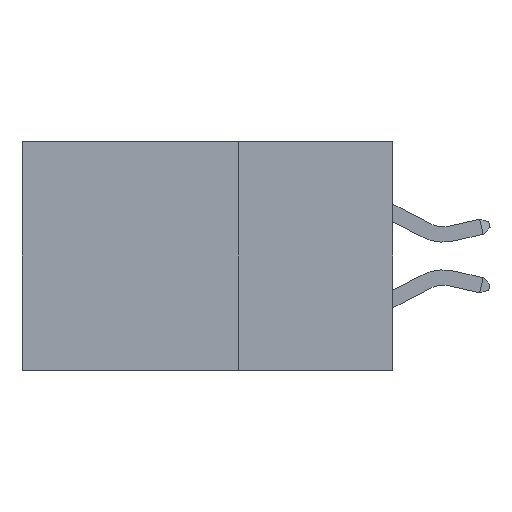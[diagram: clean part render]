
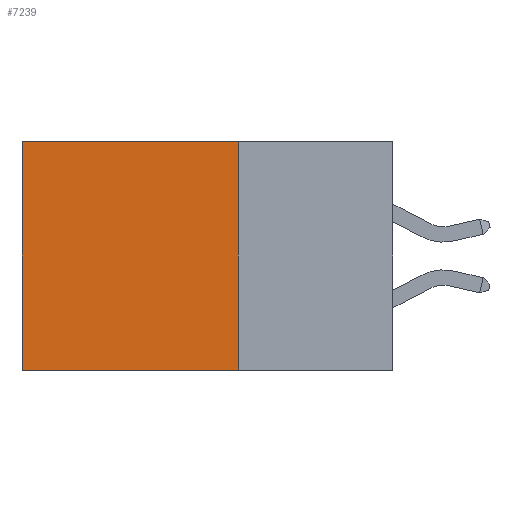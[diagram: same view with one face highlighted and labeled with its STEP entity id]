
A CAD part, left-side view. The second image highlights one B-rep face of the part: STEP entity #7239.
In plain terms, the highlighted planar face has unit normal (-1, 0, 0).
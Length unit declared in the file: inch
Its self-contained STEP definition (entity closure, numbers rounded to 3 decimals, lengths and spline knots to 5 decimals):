
#3 = DIRECTION ( 'NONE',  ( 0., 0., -1. ) ) ;
#237 = VECTOR ( 'NONE', #8397, 39.37008 ) ;
#332 = DIRECTION ( 'NONE',  ( 0., 1., 0. ) ) ;
#712 = DIRECTION ( 'NONE',  ( 0., 0., -1. ) ) ;
#816 = CARTESIAN_POINT ( 'NONE',  ( 0.2875, 0.6, -0.37 ) ) ;
#1140 = EDGE_CURVE ( 'NONE', #10898, #10252, #10301, .T. ) ;
#2216 = VECTOR ( 'NONE', #3, 39.37008 ) ;
#2453 = EDGE_CURVE ( 'NONE', #8843, #10898, #10870, .T. ) ;
#3740 = CARTESIAN_POINT ( 'NONE',  ( 0.2875, 0.25, 0. ) ) ;
#4694 = PLANE ( 'NONE',  #7935 ) ;
#4788 = CARTESIAN_POINT ( 'NONE',  ( 0.2875, 0.25, 0. ) ) ;
#5126 = CARTESIAN_POINT ( 'NONE',  ( 0.2875, 0.25, -0.37 ) ) ;
#5264 = EDGE_CURVE ( 'NONE', #8843, #10979, #7768, .T. ) ;
#5295 = CARTESIAN_POINT ( 'NONE',  ( 0.2875, 0.6, 0. ) ) ;
#5624 = DIRECTION ( 'NONE',  ( 0., 0., -1. ) ) ;
#6026 = CARTESIAN_POINT ( 'NONE',  ( 0.2875, 0.25, 0. ) ) ;
#6212 = CARTESIAN_POINT ( 'NONE',  ( 0.2875, 0.25, -0.37 ) ) ;
#7239 = ADVANCED_FACE ( 'NONE', ( #7722 ), #4694, .F. ) ;
#7722 = FACE_OUTER_BOUND ( 'NONE', #7723, .T. ) ;
#7723 = EDGE_LOOP ( 'NONE', ( #8937, #8780, #8626, #8813 ) ) ;
#7768 = LINE ( 'NONE', #8411, #237 ) ;
#7935 = AXIS2_PLACEMENT_3D ( 'NONE', #3740, #10412, #5624 ) ;
#8102 = VECTOR ( 'NONE', #332, 39.37008 ) ;
#8360 = VECTOR ( 'NONE', #712, 39.37008 ) ;
#8397 = DIRECTION ( 'NONE',  ( 0., 1., 0. ) ) ;
#8411 = CARTESIAN_POINT ( 'NONE',  ( 0.2875, 0.25, 0. ) ) ;
#8626 = ORIENTED_EDGE ( 'NONE', *, *, #2453, .F. ) ;
#8780 = ORIENTED_EDGE ( 'NONE', *, *, #1140, .F. ) ;
#8810 = LINE ( 'NONE', #5295, #8360 ) ;
#8813 = ORIENTED_EDGE ( 'NONE', *, *, #5264, .T. ) ;
#8843 = VERTEX_POINT ( 'NONE', #6026 ) ;
#8937 = ORIENTED_EDGE ( 'NONE', *, *, #10892, .T. ) ;
#10205 = CARTESIAN_POINT ( 'NONE',  ( 0.2875, 0.6, 0. ) ) ;
#10252 = VERTEX_POINT ( 'NONE', #816 ) ;
#10301 = LINE ( 'NONE', #5126, #8102 ) ;
#10412 = DIRECTION ( 'NONE',  ( 1., 0., 0. ) ) ;
#10870 = LINE ( 'NONE', #4788, #2216 ) ;
#10892 = EDGE_CURVE ( 'NONE', #10979, #10252, #8810, .T. ) ;
#10898 = VERTEX_POINT ( 'NONE', #6212 ) ;
#10979 = VERTEX_POINT ( 'NONE', #10205 ) ;
